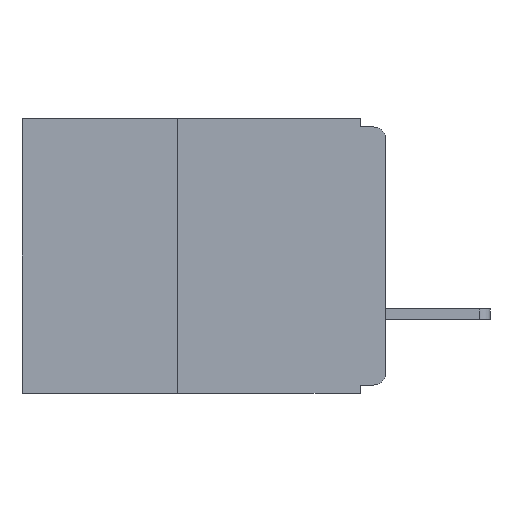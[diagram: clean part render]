
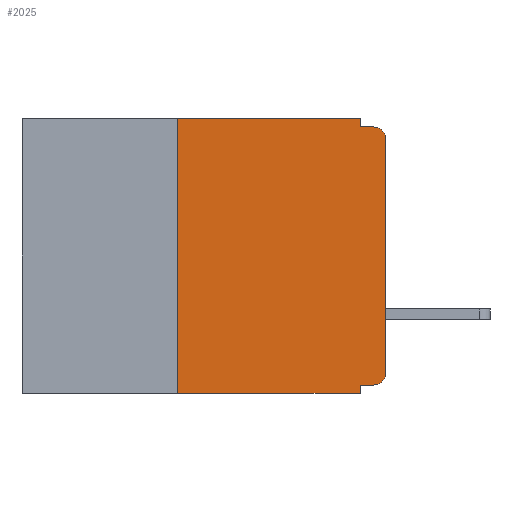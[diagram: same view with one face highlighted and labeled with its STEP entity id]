
A CAD part, left-side view. The second image highlights one B-rep face of the part: STEP entity #2025.
In plain terms, the highlighted planar face has unit normal (-1, 0, 0).
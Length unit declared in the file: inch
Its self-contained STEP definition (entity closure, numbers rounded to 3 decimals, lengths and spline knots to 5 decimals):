
#334 = CARTESIAN_POINT ( 'NONE',  ( 0., 0.25, 0. ) ) ;
#585 = LINE ( 'NONE', #5193, #13709 ) ;
#762 = VECTOR ( 'NONE', #3851, 39.37008 ) ;
#869 = VECTOR ( 'NONE', #12850, 39.37008 ) ;
#1020 = VERTEX_POINT ( 'NONE', #14104 ) ;
#1023 = CARTESIAN_POINT ( 'NONE',  ( 0., 0., 0. ) ) ;
#1054 = ORIENTED_EDGE ( 'NONE', *, *, #7827, .F. ) ;
#1089 = ORIENTED_EDGE ( 'NONE', *, *, #5577, .F. ) ;
#1177 = LINE ( 'NONE', #3798, #762 ) ;
#1506 = VECTOR ( 'NONE', #1592, 39.37008 ) ;
#1592 = DIRECTION ( 'NONE',  ( 0., 0., 1. ) ) ;
#2025 = ADVANCED_FACE ( 'NONE', ( #11908 ), #11053, .F. ) ;
#2108 = LINE ( 'NONE', #15039, #8517 ) ;
#2144 = ORIENTED_EDGE ( 'NONE', *, *, #7874, .F. ) ;
#2312 = CARTESIAN_POINT ( 'NONE',  ( 0., 0.031, 0. ) ) ;
#2570 = CARTESIAN_POINT ( 'NONE',  ( 0., 0.031, -0.01 ) ) ;
#2608 = DIRECTION ( 'NONE',  ( 0., -1., 0. ) ) ;
#2679 = ORIENTED_EDGE ( 'NONE', *, *, #5081, .T. ) ;
#3488 = AXIS2_PLACEMENT_3D ( 'NONE', #11475, #10781, #10597 ) ;
#3798 = CARTESIAN_POINT ( 'NONE',  ( 0., 0.437, -0.33 ) ) ;
#3850 = CARTESIAN_POINT ( 'NONE',  ( 0., 0.015, -0.32 ) ) ;
#3851 = DIRECTION ( 'NONE',  ( 0., -1., 0. ) ) ;
#3893 = VERTEX_POINT ( 'NONE', #8580 ) ;
#4258 = LINE ( 'NONE', #7673, #10589 ) ;
#4338 = CIRCLE ( 'NONE', #11555, 0.015 ) ;
#4358 = LINE ( 'NONE', #13217, #869 ) ;
#4384 = VERTEX_POINT ( 'NONE', #9668 ) ;
#4476 = AXIS2_PLACEMENT_3D ( 'NONE', #5736, #14439, #7006 ) ;
#5017 = ORIENTED_EDGE ( 'NONE', *, *, #7750, .F. ) ;
#5081 = EDGE_CURVE ( 'NONE', #6068, #4384, #7942, .T. ) ;
#5110 = CARTESIAN_POINT ( 'NONE',  ( 0., 0.031, 0. ) ) ;
#5193 = CARTESIAN_POINT ( 'NONE',  ( 0., 0.437, 0. ) ) ;
#5274 = EDGE_CURVE ( 'NONE', #9606, #1020, #4358, .T. ) ;
#5448 = VECTOR ( 'NONE', #8847, 39.37008 ) ;
#5577 = EDGE_CURVE ( 'NONE', #13460, #7843, #2108, .T. ) ;
#5628 = EDGE_CURVE ( 'NONE', #4384, #1020, #4338, .T. ) ;
#5736 = CARTESIAN_POINT ( 'NONE',  ( 0., 0.015, -0.305 ) ) ;
#5850 = EDGE_CURVE ( 'NONE', #13460, #6068, #7499, .T. ) ;
#5961 = ORIENTED_EDGE ( 'NONE', *, *, #7869, .T. ) ;
#6068 = VERTEX_POINT ( 'NONE', #16013 ) ;
#6580 = CARTESIAN_POINT ( 'NONE',  ( 0., 0.015, -0.025 ) ) ;
#7006 = DIRECTION ( 'NONE',  ( 0., 0., -1. ) ) ;
#7133 = ORIENTED_EDGE ( 'NONE', *, *, #5850, .T. ) ;
#7265 = ORIENTED_EDGE ( 'NONE', *, *, #7326, .F. ) ;
#7326 = EDGE_CURVE ( 'NONE', #13014, #14973, #585, .T. ) ;
#7499 = CIRCLE ( 'NONE', #4476, 0.015 ) ;
#7673 = CARTESIAN_POINT ( 'NONE',  ( 0., 0.031, -0.33 ) ) ;
#7750 = EDGE_CURVE ( 'NONE', #14973, #9606, #9608, .T. ) ;
#7827 = EDGE_CURVE ( 'NONE', #9636, #13014, #14586, .T. ) ;
#7843 = VERTEX_POINT ( 'NONE', #16054 ) ;
#7858 = DIRECTION ( 'NONE',  ( 0., 0., -1. ) ) ;
#7869 = EDGE_CURVE ( 'NONE', #9636, #3893, #1177, .T. ) ;
#7874 = EDGE_CURVE ( 'NONE', #7843, #3893, #4258, .T. ) ;
#7942 = LINE ( 'NONE', #1023, #1506 ) ;
#8517 = VECTOR ( 'NONE', #16172, 39.37008 ) ;
#8580 = CARTESIAN_POINT ( 'NONE',  ( 0., 0.031, -0.33 ) ) ;
#8847 = DIRECTION ( 'NONE',  ( 0., 0., 1. ) ) ;
#8957 = DIRECTION ( 'NONE',  ( 0., 0., -1. ) ) ;
#9035 = EDGE_LOOP ( 'NONE', ( #2679, #10825, #14617, #5017, #7265, #1054, #5961, #2144, #1089, #7133 ) ) ;
#9606 = VERTEX_POINT ( 'NONE', #2570 ) ;
#9608 = LINE ( 'NONE', #2312, #15657 ) ;
#9636 = VERTEX_POINT ( 'NONE', #13970 ) ;
#9668 = CARTESIAN_POINT ( 'NONE',  ( 0., 0., -0.025 ) ) ;
#10589 = VECTOR ( 'NONE', #8957, 39.37008 ) ;
#10597 = DIRECTION ( 'NONE',  ( 0., 0., -1. ) ) ;
#10781 = DIRECTION ( 'NONE',  ( 1., 0., 0. ) ) ;
#10825 = ORIENTED_EDGE ( 'NONE', *, *, #5628, .T. ) ;
#11053 = PLANE ( 'NONE',  #3488 ) ;
#11187 = DIRECTION ( 'NONE',  ( 0., 0., -1. ) ) ;
#11475 = CARTESIAN_POINT ( 'NONE',  ( 0., 0.437, 0. ) ) ;
#11555 = AXIS2_PLACEMENT_3D ( 'NONE', #6580, #15182, #7858 ) ;
#11908 = FACE_OUTER_BOUND ( 'NONE', #9035, .T. ) ;
#12850 = DIRECTION ( 'NONE',  ( 0., -1., 0. ) ) ;
#13014 = VERTEX_POINT ( 'NONE', #334 ) ;
#13217 = CARTESIAN_POINT ( 'NONE',  ( 0., 0., -0.01 ) ) ;
#13460 = VERTEX_POINT ( 'NONE', #3850 ) ;
#13709 = VECTOR ( 'NONE', #2608, 39.37008 ) ;
#13970 = CARTESIAN_POINT ( 'NONE',  ( 0., 0.25, -0.33 ) ) ;
#14104 = CARTESIAN_POINT ( 'NONE',  ( 0., 0.015, -0.01 ) ) ;
#14439 = DIRECTION ( 'NONE',  ( -1., 0., 0. ) ) ;
#14586 = LINE ( 'NONE', #14925, #5448 ) ;
#14617 = ORIENTED_EDGE ( 'NONE', *, *, #5274, .F. ) ;
#14925 = CARTESIAN_POINT ( 'NONE',  ( 0., 0.25, -0.33 ) ) ;
#14973 = VERTEX_POINT ( 'NONE', #5110 ) ;
#15039 = CARTESIAN_POINT ( 'NONE',  ( 0., 0., -0.32 ) ) ;
#15182 = DIRECTION ( 'NONE',  ( -1., 0., 0. ) ) ;
#15657 = VECTOR ( 'NONE', #11187, 39.37008 ) ;
#16013 = CARTESIAN_POINT ( 'NONE',  ( 0., 0., -0.305 ) ) ;
#16054 = CARTESIAN_POINT ( 'NONE',  ( 0., 0.031, -0.32 ) ) ;
#16172 = DIRECTION ( 'NONE',  ( 0., 1., 0. ) ) ;
